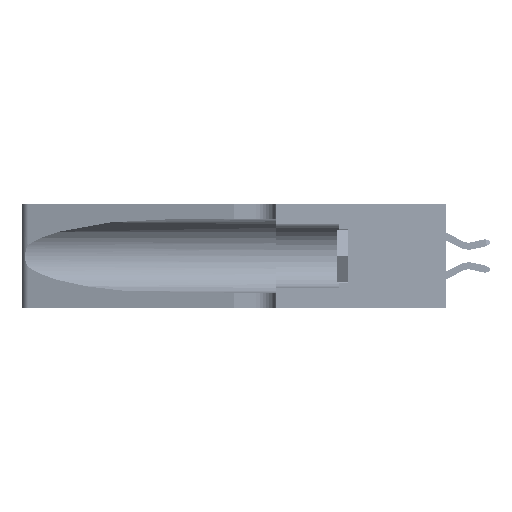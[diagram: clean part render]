
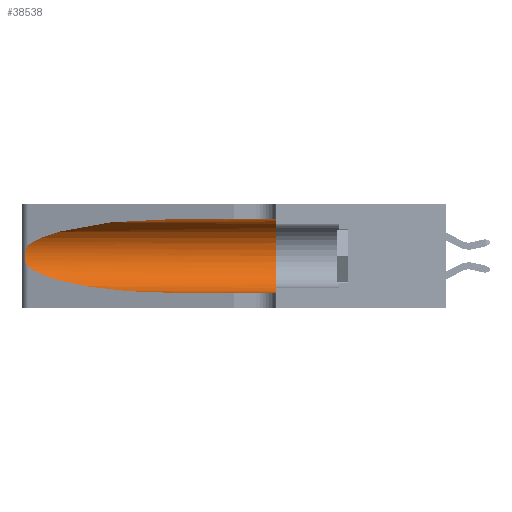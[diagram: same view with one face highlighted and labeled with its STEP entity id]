
A CAD part, left-side view. The second image highlights one B-rep face of the part: STEP entity #38538.
In plain terms, the highlighted cylindrical face has radius 3.308 mm (diameter 6.617 mm), a partial arc.
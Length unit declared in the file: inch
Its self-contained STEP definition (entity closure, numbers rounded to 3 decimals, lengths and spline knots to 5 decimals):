
#67 = CARTESIAN_POINT ( 'NONE',  ( 0.1305, 1.61858, 0.185 ) ) ;
#190 =( BOUNDED_CURVE ( )  B_SPLINE_CURVE ( 3, ( #17179, #47853, #24862, #1867 ),
 .UNSPECIFIED., .F., .F. ) 
 B_SPLINE_CURVE_WITH_KNOTS ( ( 4, 4 ),
 ( 1.5708, 2.84003 ),
 .UNSPECIFIED. ) 
 CURVE ( )  GEOMETRIC_REPRESENTATION_ITEM ( )  RATIONAL_B_SPLINE_CURVE ( ( 1., 0.87, 0.87, 1. ) ) 
 REPRESENTATION_ITEM ( '' )  );
#1867 = CARTESIAN_POINT ( 'NONE',  ( 0.25487, 1.22718, 0.22369 ) ) ;
#2001 = DIRECTION ( 'NONE',  ( 0., 1., 0. ) ) ;
#2444 = EDGE_LOOP ( 'NONE', ( #6561, #9693, #37855, #17341, #4779, #41997 ) ) ;
#3308 = CARTESIAN_POINT ( 'NONE',  ( 0.25639, 1.23184, 0.21858 ) ) ;
#4779 = ORIENTED_EDGE ( 'NONE', *, *, #28640, .F. ) ;
#6561 = ORIENTED_EDGE ( 'NONE', *, *, #26814, .T. ) ;
#6774 = LINE ( 'NONE', #46834, #25988 ) ;
#7161 = CARTESIAN_POINT ( 'NONE',  ( 0.25854, 1.2359, 0.20912 ) ) ;
#7521 = CARTESIAN_POINT ( 'NONE',  ( 0.1305, 1.61858, 0.31525 ) ) ;
#7585 = DIRECTION ( 'NONE',  ( 0., 0., -1. ) ) ;
#8991 = CARTESIAN_POINT ( 'NONE',  ( 0.18966, 0.96281, 0.05475 ) ) ;
#9476 = CARTESIAN_POINT ( 'NONE',  ( 0.25487, 1.22718, 0.22369 ) ) ;
#9693 = ORIENTED_EDGE ( 'NONE', *, *, #30542, .T. ) ;
#9789 = VERTEX_POINT ( 'NONE', #35478 ) ;
#10398 = CARTESIAN_POINT ( 'NONE',  ( 0.1305, 0.72297, 0.05475 ) ) ;
#11030 = CARTESIAN_POINT ( 'NONE',  ( 0.26075, 1.23896, 0.19203 ) ) ;
#13905 = VERTEX_POINT ( 'NONE', #26105 ) ;
#14704 = CARTESIAN_POINT ( 'NONE',  ( 0.25487, 1.22718, 0.14631 ) ) ;
#14926 = CARTESIAN_POINT ( 'NONE',  ( 0.26017, 1.23833, 0.17102 ) ) ;
#15896 = CARTESIAN_POINT ( 'NONE',  ( 0.1305, 0.35, 0.05475 ) ) ;
#17179 = CARTESIAN_POINT ( 'NONE',  ( 0.1305, 0.72297, 0.31525 ) ) ;
#17341 = ORIENTED_EDGE ( 'NONE', *, *, #28439, .T. ) ;
#18600 = CARTESIAN_POINT ( 'NONE',  ( 0.25555, 1.22994, 0.2215 ) ) ;
#18758 = CARTESIAN_POINT ( 'NONE',  ( 0.25789, 1.23486, 0.15765 ) ) ;
#21364 = EDGE_CURVE ( 'NONE', #42928, #33802, #23231, .T. ) ;
#21840 = AXIS2_PLACEMENT_3D ( 'NONE', #24993, #2001, #28845 ) ;
#22594 = CARTESIAN_POINT ( 'NONE',  ( 0.25555, 1.22993, 0.14849 ) ) ;
#23231 =( BOUNDED_CURVE ( )  B_SPLINE_CURVE ( 3, ( #31948, #35835, #8991, #39731 ),
 .UNSPECIFIED., .F., .F. ) 
 B_SPLINE_CURVE_WITH_KNOTS ( ( 4, 4 ),
 ( 3.44316, 4.71239 ),
 .UNSPECIFIED. ) 
 CURVE ( )  GEOMETRIC_REPRESENTATION_ITEM ( )  RATIONAL_B_SPLINE_CURVE ( ( 1., 0.87, 0.87, 1. ) ) 
 REPRESENTATION_ITEM ( '' )  );
#24862 = CARTESIAN_POINT ( 'NONE',  ( 0.2373, 1.15595, 0.28018 ) ) ;
#24993 = CARTESIAN_POINT ( 'NONE',  ( 0.1305, 0.35, 0.185 ) ) ;
#25988 = VECTOR ( 'NONE', #31527, 39.37008 ) ;
#26105 = CARTESIAN_POINT ( 'NONE',  ( 0.1305, 0.72297, 0.31525 ) ) ;
#26814 = EDGE_CURVE ( 'NONE', #13905, #40482, #190, .T. ) ;
#26889 = DIRECTION ( 'NONE',  ( 0., -1., 0. ) ) ;
#28439 = EDGE_CURVE ( 'NONE', #33802, #45063, #6774, .T. ) ;
#28538 = FACE_OUTER_BOUND ( 'NONE', #2444, .T. ) ;
#28640 = EDGE_CURVE ( 'NONE', #9789, #45063, #42749, .T. ) ;
#28845 = DIRECTION ( 'NONE',  ( 0., 0., 1. ) ) ;
#30136 = CARTESIAN_POINT ( 'NONE',  ( 0.25787, 1.23484, 0.2124 ) ) ;
#30542 = EDGE_CURVE ( 'NONE', #40482, #42928, #38174, .T. ) ;
#31527 = DIRECTION ( 'NONE',  ( 0., -1., 0. ) ) ;
#31948 = CARTESIAN_POINT ( 'NONE',  ( 0.25487, 1.22718, 0.14631 ) ) ;
#33802 = VERTEX_POINT ( 'NONE', #10398 ) ;
#33986 = EDGE_CURVE ( 'NONE', #13905, #9789, #45238, .T. ) ;
#33993 = CARTESIAN_POINT ( 'NONE',  ( 0.26018, 1.23835, 0.19895 ) ) ;
#35000 = VECTOR ( 'NONE', #38276, 39.37008 ) ;
#35478 = CARTESIAN_POINT ( 'NONE',  ( 0.1305, 0.35, 0.31525 ) ) ;
#35835 = CARTESIAN_POINT ( 'NONE',  ( 0.2373, 1.15595, 0.08982 ) ) ;
#35971 = AXIS2_PLACEMENT_3D ( 'NONE', #67, #26889, #7585 ) ;
#37855 = ORIENTED_EDGE ( 'NONE', *, *, #21364, .T. ) ;
#37908 = CARTESIAN_POINT ( 'NONE',  ( 0.26075, 1.23896, 0.178 ) ) ;
#38174 = B_SPLINE_CURVE_WITH_KNOTS ( 'NONE', 3,
 ( #49280, #18600, #3308, #30136, #7161, #33993, #11030, #37908, #14926, #41771, #18758, #45599, #22594, #49439 ),
 .UNSPECIFIED., .F., .F.,
 ( 4, 2, 2, 2, 2, 2, 4 ),
 ( 0., 0.00027, 0.00053, 0.00107, 0.0016, 0.00187, 0.00214 ),
 .UNSPECIFIED. ) ;
#38276 = DIRECTION ( 'NONE',  ( 0., -1., 0. ) ) ;
#38538 = ADVANCED_FACE ( 'NONE', ( #28538 ), #47773, .F. ) ;
#39731 = CARTESIAN_POINT ( 'NONE',  ( 0.1305, 0.72297, 0.05475 ) ) ;
#40482 = VERTEX_POINT ( 'NONE', #9476 ) ;
#41771 = CARTESIAN_POINT ( 'NONE',  ( 0.25856, 1.23593, 0.16098 ) ) ;
#41997 = ORIENTED_EDGE ( 'NONE', *, *, #33986, .F. ) ;
#42749 = CIRCLE ( 'NONE', #21840, 0.13025 ) ;
#42928 = VERTEX_POINT ( 'NONE', #14704 ) ;
#45063 = VERTEX_POINT ( 'NONE', #15896 ) ;
#45238 = LINE ( 'NONE', #7521, #35000 ) ;
#45599 = CARTESIAN_POINT ( 'NONE',  ( 0.25639, 1.23186, 0.15144 ) ) ;
#46834 = CARTESIAN_POINT ( 'NONE',  ( 0.1305, 1.61858, 0.05475 ) ) ;
#47773 = CYLINDRICAL_SURFACE ( 'NONE', #35971, 0.13025 ) ;
#47853 = CARTESIAN_POINT ( 'NONE',  ( 0.18966, 0.96281, 0.31525 ) ) ;
#49280 = CARTESIAN_POINT ( 'NONE',  ( 0.25487, 1.22718, 0.22369 ) ) ;
#49439 = CARTESIAN_POINT ( 'NONE',  ( 0.25487, 1.22718, 0.14631 ) ) ;
